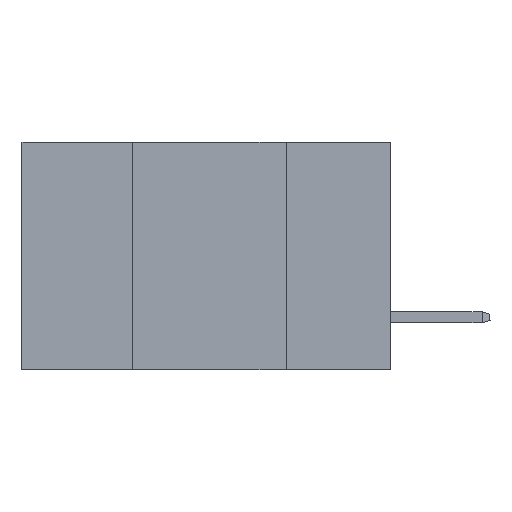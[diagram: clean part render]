
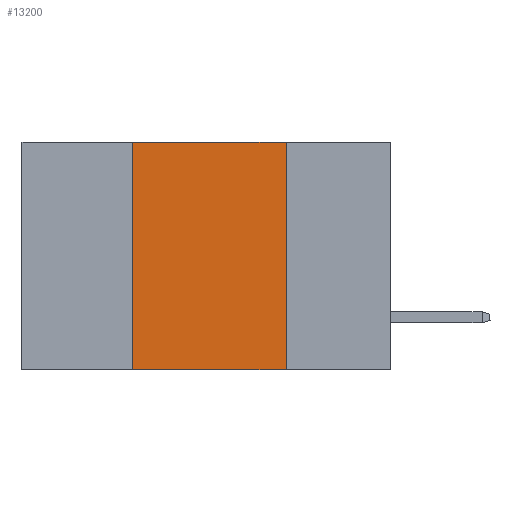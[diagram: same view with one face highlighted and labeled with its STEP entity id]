
A CAD part, left-side view. The second image highlights one B-rep face of the part: STEP entity #13200.
In plain terms, the highlighted planar face has unit normal (-1, 0, 0).
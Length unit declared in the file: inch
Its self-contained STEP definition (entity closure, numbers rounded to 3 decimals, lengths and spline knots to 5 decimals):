
#690 = VECTOR ( 'NONE', #2030, 39.37008 ) ;
#2030 = DIRECTION ( 'NONE',  ( 0., 0., 1. ) ) ;
#2610 = DIRECTION ( 'NONE',  ( 0., -1., 0. ) ) ;
#3855 = EDGE_CURVE ( 'NONE', #6002, #22924, #4887, .T. ) ;
#3945 = CARTESIAN_POINT ( 'NONE',  ( 0., 0.42, -0.37 ) ) ;
#4887 = LINE ( 'NONE', #25481, #690 ) ;
#5599 = PLANE ( 'NONE',  #16934 ) ;
#5909 = CARTESIAN_POINT ( 'NONE',  ( 0., 0.6, -0.37 ) ) ;
#6002 = VERTEX_POINT ( 'NONE', #3945 ) ;
#7397 = EDGE_CURVE ( 'NONE', #6002, #13182, #22551, .T. ) ;
#8257 = CARTESIAN_POINT ( 'NONE',  ( 0., 0.6, 0. ) ) ;
#9478 = ORIENTED_EDGE ( 'NONE', *, *, #7397, .T. ) ;
#10643 = LINE ( 'NONE', #20270, #37098 ) ;
#13182 = VERTEX_POINT ( 'NONE', #22469 ) ;
#13200 = ADVANCED_FACE ( 'NONE', ( #35652 ), #5599, .F. ) ;
#15164 = EDGE_CURVE ( 'NONE', #22924, #23663, #17155, .T. ) ;
#16934 = AXIS2_PLACEMENT_3D ( 'NONE', #8257, #32140, #21609 ) ;
#17155 = LINE ( 'NONE', #30549, #43015 ) ;
#17536 = ORIENTED_EDGE ( 'NONE', *, *, #42831, .F. ) ;
#20270 = CARTESIAN_POINT ( 'NONE',  ( 0., 0.17, 0. ) ) ;
#21609 = DIRECTION ( 'NONE',  ( 0., 0., -1. ) ) ;
#22344 = EDGE_LOOP ( 'NONE', ( #17536, #37278, #24985, #9478 ) ) ;
#22469 = CARTESIAN_POINT ( 'NONE',  ( 0., 0.17, -0.37 ) ) ;
#22551 = LINE ( 'NONE', #5909, #28952 ) ;
#22924 = VERTEX_POINT ( 'NONE', #25068 ) ;
#23663 = VERTEX_POINT ( 'NONE', #23914 ) ;
#23914 = CARTESIAN_POINT ( 'NONE',  ( 0., 0.17, 0. ) ) ;
#24985 = ORIENTED_EDGE ( 'NONE', *, *, #3855, .F. ) ;
#25068 = CARTESIAN_POINT ( 'NONE',  ( 0., 0.42, 0. ) ) ;
#25481 = CARTESIAN_POINT ( 'NONE',  ( 0., 0.42, 0. ) ) ;
#28952 = VECTOR ( 'NONE', #2610, 39.37008 ) ;
#30549 = CARTESIAN_POINT ( 'NONE',  ( 0., 0.6, 0. ) ) ;
#32140 = DIRECTION ( 'NONE',  ( 1., 0., 0. ) ) ;
#35652 = FACE_OUTER_BOUND ( 'NONE', #22344, .T. ) ;
#37098 = VECTOR ( 'NONE', #39818, 39.37008 ) ;
#37278 = ORIENTED_EDGE ( 'NONE', *, *, #15164, .F. ) ;
#39818 = DIRECTION ( 'NONE',  ( 0., 0., -1. ) ) ;
#40635 = DIRECTION ( 'NONE',  ( 0., -1., 0. ) ) ;
#42831 = EDGE_CURVE ( 'NONE', #23663, #13182, #10643, .T. ) ;
#43015 = VECTOR ( 'NONE', #40635, 39.37008 ) ;
